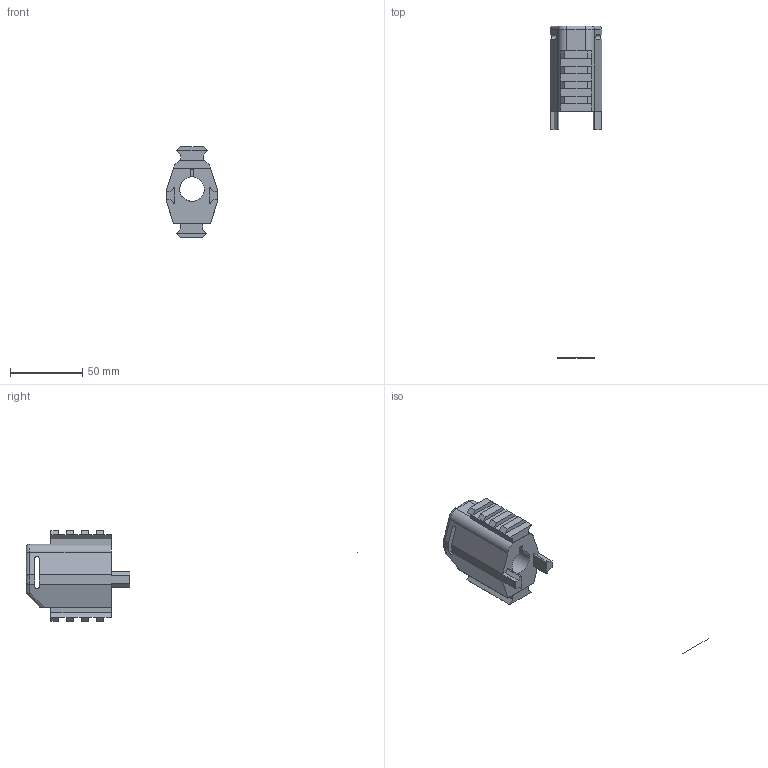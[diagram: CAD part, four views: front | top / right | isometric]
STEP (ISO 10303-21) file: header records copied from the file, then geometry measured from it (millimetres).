
FILE_DESCRIPTION(/* description */ (''),/* implementation_level */ '2;1');
FILE_NAME(/* name */ 'HRR PRA - 6in Endcap v5.step',/* time_stamp */ '2020-03-16T00:15:39-04:00',/* author */ (''),/* organization */ (''),/* preprocessor_version */ 'ST-DEVELOPER v18',/* originating_system */ 'Autodesk Translation Framework v8.12.0.6',/* authorisation */ '');
FILE_SCHEMA (('AUTOMOTIVE_DESIGN { 1 0 10303 214 3 1 1 }'));
Length unit declared in the file: millimetre
Products named in the file (1): HRR PRA - 6in Endcap
Bounding box: 35.56 x 229.61 x 62.84 mm (x, y, z)
Volume: 73884.1 mm3; surface area: 20783.3 mm2
Topology: 4 solids, 4 shells, 121 faces, 325 edges, 210 vertices
Faces by surface type: plane 96, cylinder 20, bspline 2, torus 2, cone 1
Full cylindrical faces by diameter (mm): 17 x2
Entity records: 3791 total; most frequent: CARTESIAN_POINT 693, ORIENTED_EDGE 650, DIRECTION 609, EDGE_CURVE 325, LINE 277, VECTOR 277, VERTEX_POINT 210, AXIS2_PLACEMENT_3D 166
